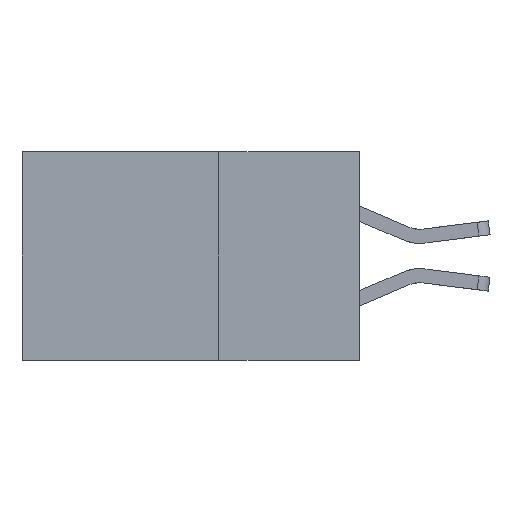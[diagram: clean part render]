
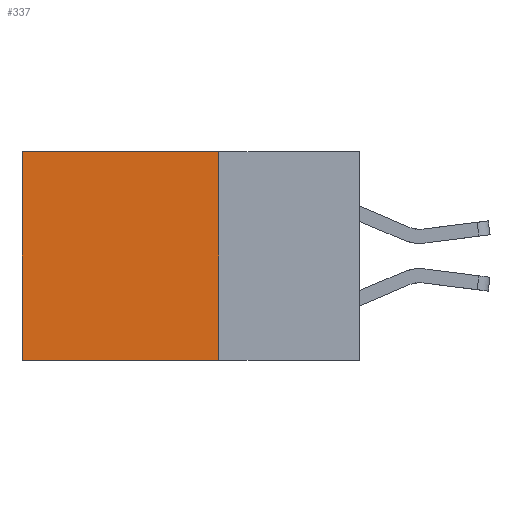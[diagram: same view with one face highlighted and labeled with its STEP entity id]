
A CAD part, left-side view. The second image highlights one B-rep face of the part: STEP entity #337.
In plain terms, the highlighted planar face has unit normal (-1, 0, 0).
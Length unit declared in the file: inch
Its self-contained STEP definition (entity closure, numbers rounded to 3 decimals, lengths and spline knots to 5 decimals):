
#68 = EDGE_CURVE ( 'NONE', #3035, #11023, #7705, .T. ) ;
#103 = EDGE_LOOP ( 'NONE', ( #6118, #2893, #5027, #5749 ) ) ;
#276 = FACE_OUTER_BOUND ( 'NONE', #103, .T. ) ;
#337 = ADVANCED_FACE ( 'NONE', ( #276 ), #10874, .F. ) ;
#404 = LINE ( 'NONE', #10631, #944 ) ;
#944 = VECTOR ( 'NONE', #9094, 39.37008 ) ;
#985 = CARTESIAN_POINT ( 'NONE',  ( 0.2875, 0.25, 0. ) ) ;
#1755 = VECTOR ( 'NONE', #8756, 39.37008 ) ;
#2893 = ORIENTED_EDGE ( 'NONE', *, *, #5758, .F. ) ;
#3035 = VERTEX_POINT ( 'NONE', #6132 ) ;
#3253 = EDGE_CURVE ( 'NONE', #3035, #4169, #404, .T. ) ;
#3550 = VECTOR ( 'NONE', #5649, 39.37008 ) ;
#3693 = CARTESIAN_POINT ( 'NONE',  ( 0.2875, 0.25, -0.37 ) ) ;
#3788 = DIRECTION ( 'NONE',  ( 0., 0., -1. ) ) ;
#3936 = CARTESIAN_POINT ( 'NONE',  ( 0.2875, 0.6, 0. ) ) ;
#4169 = VERTEX_POINT ( 'NONE', #3693 ) ;
#5027 = ORIENTED_EDGE ( 'NONE', *, *, #3253, .F. ) ;
#5035 = DIRECTION ( 'NONE',  ( 0., 0., -1. ) ) ;
#5488 = LINE ( 'NONE', #3936, #11204 ) ;
#5649 = DIRECTION ( 'NONE',  ( 0., 1., 0. ) ) ;
#5720 = CARTESIAN_POINT ( 'NONE',  ( 0.2875, 0.25, 0. ) ) ;
#5749 = ORIENTED_EDGE ( 'NONE', *, *, #68, .T. ) ;
#5758 = EDGE_CURVE ( 'NONE', #4169, #8999, #10597, .T. ) ;
#6118 = ORIENTED_EDGE ( 'NONE', *, *, #10610, .T. ) ;
#6132 = CARTESIAN_POINT ( 'NONE',  ( 0.2875, 0.25, 0. ) ) ;
#6693 = DIRECTION ( 'NONE',  ( 1., 0., 0. ) ) ;
#7365 = CARTESIAN_POINT ( 'NONE',  ( 0.2875, 0.6, 0. ) ) ;
#7372 = AXIS2_PLACEMENT_3D ( 'NONE', #5720, #6693, #5035 ) ;
#7705 = LINE ( 'NONE', #985, #1755 ) ;
#8222 = CARTESIAN_POINT ( 'NONE',  ( 0.2875, 0.25, -0.37 ) ) ;
#8756 = DIRECTION ( 'NONE',  ( 0., 1., 0. ) ) ;
#8824 = CARTESIAN_POINT ( 'NONE',  ( 0.2875, 0.6, -0.37 ) ) ;
#8999 = VERTEX_POINT ( 'NONE', #8824 ) ;
#9094 = DIRECTION ( 'NONE',  ( 0., 0., -1. ) ) ;
#10597 = LINE ( 'NONE', #8222, #3550 ) ;
#10610 = EDGE_CURVE ( 'NONE', #11023, #8999, #5488, .T. ) ;
#10631 = CARTESIAN_POINT ( 'NONE',  ( 0.2875, 0.25, 0. ) ) ;
#10874 = PLANE ( 'NONE',  #7372 ) ;
#11023 = VERTEX_POINT ( 'NONE', #7365 ) ;
#11204 = VECTOR ( 'NONE', #3788, 39.37008 ) ;
